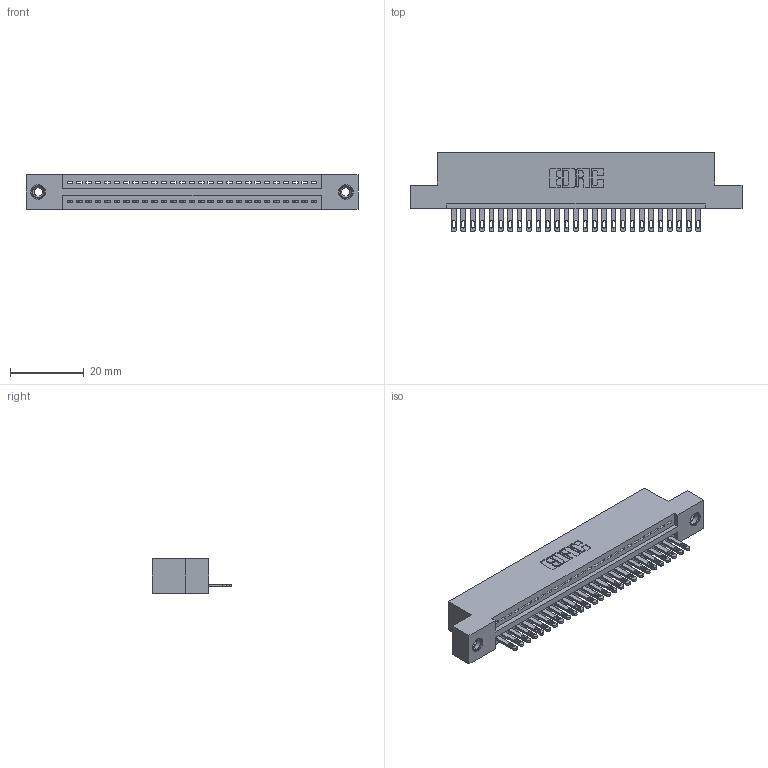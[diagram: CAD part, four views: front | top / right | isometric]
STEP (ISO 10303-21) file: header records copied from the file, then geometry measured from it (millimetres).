
FILE_DESCRIPTION (( 'STEP AP203' ), '1' );
FILE_NAME ('345-027-500-108.STEP', '2018-08-22T04:32:17', ( '' ), ( '' ), 'SwSTEP 2.0', 'SolidWorks 2016', '' );
FILE_SCHEMA (( 'CONFIG_CONTROL_DESIGN' ));
Length unit declared in the file: inch
Products named in the file (4): 345 Part_Flush Mounting Lugs - 0.156 Dia-TI; 345-292-001_345-293-100; 345-250-001_345-250-003-102; 345-027-500-108
Assembly tree (30 placements, depth 2):
  345-027-500-108
    345 Part_Flush Mounting Lugs - 0.156 Dia-TI
    345-292-001_345-293-100  x27
    345-250-001_345-250-003-102  x2
Bounding box: 89.79 x 21.51 x 9.4 mm (x, y, z)
Volume: 8415.6 mm3; surface area: 11059.5 mm2
Topology: 30 solids, 30 shells, 1644 faces, 5013 edges, 3334 vertices
Faces by surface type: plane 1030, cylinder 598, cone 12, torus 4
Entity records: 23456 total; most frequent: CARTESIAN_POINT 4044, ORIENTED_EDGE 3998, DIRECTION 3583, EDGE_CURVE 1999, VECTOR 1735, LINE 1735, VERTEX_POINT 1328, AXIS2_PLACEMENT_3D 924
